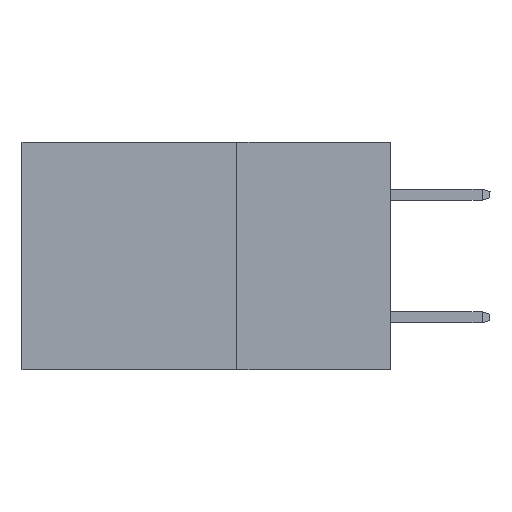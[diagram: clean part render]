
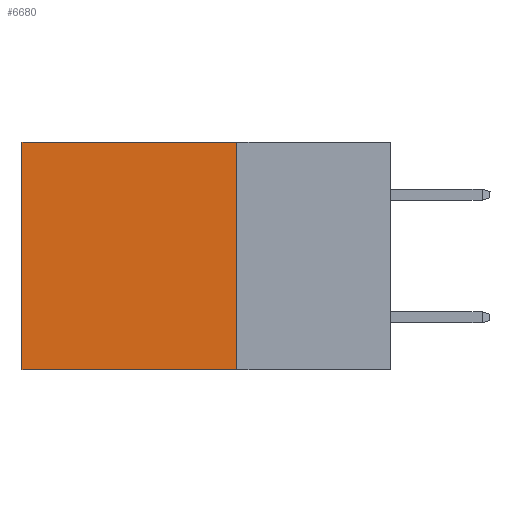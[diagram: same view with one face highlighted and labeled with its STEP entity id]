
A CAD part, left-side view. The second image highlights one B-rep face of the part: STEP entity #6680.
In plain terms, the highlighted planar face has unit normal (-1, 0, 0).
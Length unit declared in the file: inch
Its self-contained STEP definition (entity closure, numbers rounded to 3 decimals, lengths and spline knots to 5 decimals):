
#1282 = DIRECTION ( 'NONE',  ( 1., 0., 0. ) ) ;
#1565 = LINE ( 'NONE', #3631, #6503 ) ;
#1778 = CARTESIAN_POINT ( 'NONE',  ( 0.2875, 0.25, 0. ) ) ;
#2310 = CARTESIAN_POINT ( 'NONE',  ( 0.2875, 0.25, 0. ) ) ;
#2635 = DIRECTION ( 'NONE',  ( 0., 1., 0. ) ) ;
#3273 = EDGE_CURVE ( 'NONE', #11409, #9039, #1565, .T. ) ;
#3549 = LINE ( 'NONE', #9032, #4731 ) ;
#3631 = CARTESIAN_POINT ( 'NONE',  ( 0.2875, 0.6, 0. ) ) ;
#4170 = ORIENTED_EDGE ( 'NONE', *, *, #5037, .F. ) ;
#4702 = CARTESIAN_POINT ( 'NONE',  ( 0.2875, 0.6, 0. ) ) ;
#4731 = VECTOR ( 'NONE', #9999, 39.37008 ) ;
#4864 = ORIENTED_EDGE ( 'NONE', *, *, #3273, .T. ) ;
#4926 = EDGE_CURVE ( 'NONE', #5120, #9039, #6469, .T. ) ;
#5037 = EDGE_CURVE ( 'NONE', #7551, #5120, #3549, .T. ) ;
#5104 = VECTOR ( 'NONE', #2635, 39.37008 ) ;
#5120 = VERTEX_POINT ( 'NONE', #11212 ) ;
#5494 = CARTESIAN_POINT ( 'NONE',  ( 0.2875, 0.25, -0.37 ) ) ;
#5840 = DIRECTION ( 'NONE',  ( 0., 0., -1. ) ) ;
#5899 = FACE_OUTER_BOUND ( 'NONE', #6043, .T. ) ;
#6043 = EDGE_LOOP ( 'NONE', ( #4864, #10280, #4170, #10636 ) ) ;
#6469 = LINE ( 'NONE', #5494, #10565 ) ;
#6503 = VECTOR ( 'NONE', #8074, 39.37008 ) ;
#6680 = ADVANCED_FACE ( 'NONE', ( #5899 ), #6753, .F. ) ;
#6753 = PLANE ( 'NONE',  #9082 ) ;
#7551 = VERTEX_POINT ( 'NONE', #7576 ) ;
#7576 = CARTESIAN_POINT ( 'NONE',  ( 0.2875, 0.25, 0. ) ) ;
#8074 = DIRECTION ( 'NONE',  ( 0., 0., -1. ) ) ;
#9032 = CARTESIAN_POINT ( 'NONE',  ( 0.2875, 0.25, 0. ) ) ;
#9039 = VERTEX_POINT ( 'NONE', #11947 ) ;
#9082 = AXIS2_PLACEMENT_3D ( 'NONE', #2310, #1282, #5840 ) ;
#9999 = DIRECTION ( 'NONE',  ( 0., 0., -1. ) ) ;
#10110 = LINE ( 'NONE', #1778, #5104 ) ;
#10280 = ORIENTED_EDGE ( 'NONE', *, *, #4926, .F. ) ;
#10565 = VECTOR ( 'NONE', #11034, 39.37008 ) ;
#10636 = ORIENTED_EDGE ( 'NONE', *, *, #11673, .T. ) ;
#11034 = DIRECTION ( 'NONE',  ( 0., 1., 0. ) ) ;
#11212 = CARTESIAN_POINT ( 'NONE',  ( 0.2875, 0.25, -0.37 ) ) ;
#11409 = VERTEX_POINT ( 'NONE', #4702 ) ;
#11673 = EDGE_CURVE ( 'NONE', #7551, #11409, #10110, .T. ) ;
#11947 = CARTESIAN_POINT ( 'NONE',  ( 0.2875, 0.6, -0.37 ) ) ;
